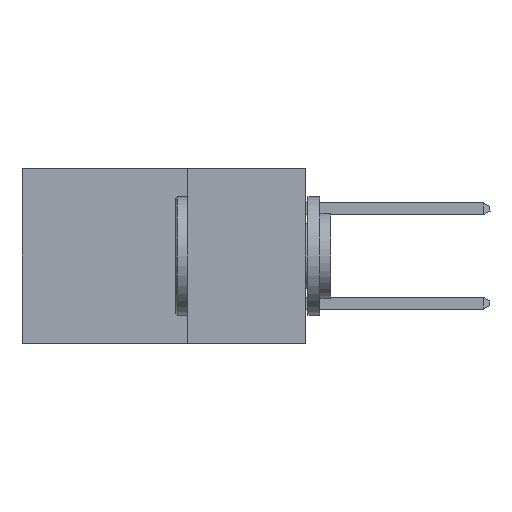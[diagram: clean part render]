
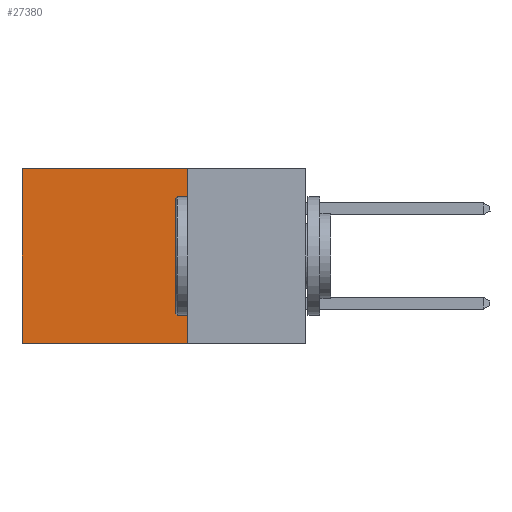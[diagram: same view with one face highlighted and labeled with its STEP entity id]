
A CAD part, left-side view. The second image highlights one B-rep face of the part: STEP entity #27380.
In plain terms, the highlighted planar face has unit normal (-1, 0, 0).
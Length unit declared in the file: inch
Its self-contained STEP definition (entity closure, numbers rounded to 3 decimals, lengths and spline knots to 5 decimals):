
#186 = VERTEX_POINT ( 'NONE', #16820 ) ;
#636 = VECTOR ( 'NONE', #26219, 39.37008 ) ;
#936 = LINE ( 'NONE', #21662, #24790 ) ;
#3675 = LINE ( 'NONE', #25244, #6612 ) ;
#4202 = CARTESIAN_POINT ( 'NONE',  ( 0.298, 0.25, -0.37 ) ) ;
#5463 = ORIENTED_EDGE ( 'NONE', *, *, #18751, .T. ) ;
#6176 = VERTEX_POINT ( 'NONE', #4202 ) ;
#6488 = VECTOR ( 'NONE', #27054, 39.37008 ) ;
#6612 = VECTOR ( 'NONE', #18982, 39.37008 ) ;
#6847 = VERTEX_POINT ( 'NONE', #9083 ) ;
#7322 = CARTESIAN_POINT ( 'NONE',  ( 0.298, 0.6, 0. ) ) ;
#7761 = ORIENTED_EDGE ( 'NONE', *, *, #19392, .F. ) ;
#8946 = DIRECTION ( 'NONE',  ( 0., 0., -1. ) ) ;
#9029 = CARTESIAN_POINT ( 'NONE',  ( 0.298, 0.6, 0. ) ) ;
#9083 = CARTESIAN_POINT ( 'NONE',  ( 0.298, 0.6, -0.37 ) ) ;
#9206 = EDGE_LOOP ( 'NONE', ( #5463, #15314, #7761, #18473 ) ) ;
#9959 = CARTESIAN_POINT ( 'NONE',  ( 0.298, 0.25, 0. ) ) ;
#12130 = LINE ( 'NONE', #12366, #6488 ) ;
#12366 = CARTESIAN_POINT ( 'NONE',  ( 0.298, 0.25, -0.37 ) ) ;
#14322 = VERTEX_POINT ( 'NONE', #7322 ) ;
#15314 = ORIENTED_EDGE ( 'NONE', *, *, #17346, .F. ) ;
#16425 = DIRECTION ( 'NONE',  ( 0., 0., -1. ) ) ;
#16820 = CARTESIAN_POINT ( 'NONE',  ( 0.298, 0.25, 0. ) ) ;
#17346 = EDGE_CURVE ( 'NONE', #6176, #6847, #12130, .T. ) ;
#17572 = LINE ( 'NONE', #9029, #636 ) ;
#17808 = FACE_OUTER_BOUND ( 'NONE', #9206, .T. ) ;
#18473 = ORIENTED_EDGE ( 'NONE', *, *, #23956, .T. ) ;
#18751 = EDGE_CURVE ( 'NONE', #14322, #6847, #17572, .T. ) ;
#18982 = DIRECTION ( 'NONE',  ( 0., 1., 0. ) ) ;
#19392 = EDGE_CURVE ( 'NONE', #186, #6176, #936, .T. ) ;
#19909 = AXIS2_PLACEMENT_3D ( 'NONE', #9959, #26976, #16425 ) ;
#20566 = PLANE ( 'NONE',  #19909 ) ;
#21662 = CARTESIAN_POINT ( 'NONE',  ( 0.298, 0.25, 0. ) ) ;
#23956 = EDGE_CURVE ( 'NONE', #186, #14322, #3675, .T. ) ;
#24790 = VECTOR ( 'NONE', #8946, 39.37008 ) ;
#25244 = CARTESIAN_POINT ( 'NONE',  ( 0.298, 0.25, 0. ) ) ;
#26219 = DIRECTION ( 'NONE',  ( 0., 0., -1. ) ) ;
#26976 = DIRECTION ( 'NONE',  ( 1., 0., 0. ) ) ;
#27054 = DIRECTION ( 'NONE',  ( 0., 1., 0. ) ) ;
#27380 = ADVANCED_FACE ( 'NONE', ( #17808 ), #20566, .F. ) ;
